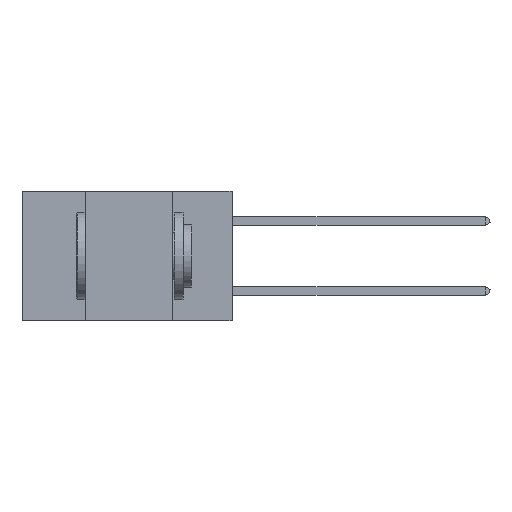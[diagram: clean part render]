
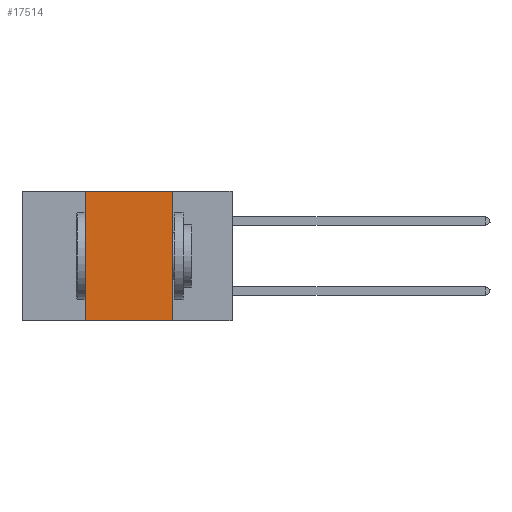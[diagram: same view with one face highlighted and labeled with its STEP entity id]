
A CAD part, left-side view. The second image highlights one B-rep face of the part: STEP entity #17514.
In plain terms, the highlighted planar face has unit normal (-1, 0, 0).
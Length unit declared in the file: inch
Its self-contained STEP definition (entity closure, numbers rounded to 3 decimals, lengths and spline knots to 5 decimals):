
#767 = CARTESIAN_POINT ( 'NONE',  ( 0., 0.6, -0.37 ) ) ;
#949 = PLANE ( 'NONE',  #9597 ) ;
#2047 = LINE ( 'NONE', #10956, #11977 ) ;
#2414 = DIRECTION ( 'NONE',  ( 0., -1., 0. ) ) ;
#3296 = CARTESIAN_POINT ( 'NONE',  ( 0., 0.6, 0. ) ) ;
#3727 = VERTEX_POINT ( 'NONE', #5237 ) ;
#5237 = CARTESIAN_POINT ( 'NONE',  ( 0., 0.17, 0. ) ) ;
#8447 = LINE ( 'NONE', #12970, #22253 ) ;
#9375 = EDGE_LOOP ( 'NONE', ( #22104, #11364, #21388, #17267 ) ) ;
#9597 = AXIS2_PLACEMENT_3D ( 'NONE', #10130, #22656, #20847 ) ;
#9637 = VERTEX_POINT ( 'NONE', #14547 ) ;
#9819 = EDGE_CURVE ( 'NONE', #12803, #9637, #20604, .T. ) ;
#10130 = CARTESIAN_POINT ( 'NONE',  ( 0., 0.6, 0. ) ) ;
#10570 = EDGE_CURVE ( 'NONE', #12803, #15169, #8447, .T. ) ;
#10956 = CARTESIAN_POINT ( 'NONE',  ( 0., 0.17, 0. ) ) ;
#11364 = ORIENTED_EDGE ( 'NONE', *, *, #21829, .F. ) ;
#11977 = VECTOR ( 'NONE', #19710, 39.37008 ) ;
#12161 = VECTOR ( 'NONE', #2414, 39.37008 ) ;
#12803 = VERTEX_POINT ( 'NONE', #17050 ) ;
#12970 = CARTESIAN_POINT ( 'NONE',  ( 0., 0.42, 0. ) ) ;
#13770 = EDGE_CURVE ( 'NONE', #3727, #9637, #2047, .T. ) ;
#14547 = CARTESIAN_POINT ( 'NONE',  ( 0., 0.17, -0.37 ) ) ;
#15169 = VERTEX_POINT ( 'NONE', #16496 ) ;
#16496 = CARTESIAN_POINT ( 'NONE',  ( 0., 0.42, 0. ) ) ;
#17050 = CARTESIAN_POINT ( 'NONE',  ( 0., 0.42, -0.37 ) ) ;
#17179 = VECTOR ( 'NONE', #17762, 39.37008 ) ;
#17267 = ORIENTED_EDGE ( 'NONE', *, *, #9819, .T. ) ;
#17514 = ADVANCED_FACE ( 'NONE', ( #23013 ), #949, .F. ) ;
#17762 = DIRECTION ( 'NONE',  ( 0., -1., 0. ) ) ;
#18961 = DIRECTION ( 'NONE',  ( 0., 0., 1. ) ) ;
#19710 = DIRECTION ( 'NONE',  ( 0., 0., -1. ) ) ;
#20604 = LINE ( 'NONE', #767, #12161 ) ;
#20847 = DIRECTION ( 'NONE',  ( 0., 0., -1. ) ) ;
#21388 = ORIENTED_EDGE ( 'NONE', *, *, #10570, .F. ) ;
#21829 = EDGE_CURVE ( 'NONE', #15169, #3727, #21954, .T. ) ;
#21954 = LINE ( 'NONE', #3296, #17179 ) ;
#22104 = ORIENTED_EDGE ( 'NONE', *, *, #13770, .F. ) ;
#22253 = VECTOR ( 'NONE', #18961, 39.37008 ) ;
#22656 = DIRECTION ( 'NONE',  ( 1., 0., 0. ) ) ;
#23013 = FACE_OUTER_BOUND ( 'NONE', #9375, .T. ) ;
